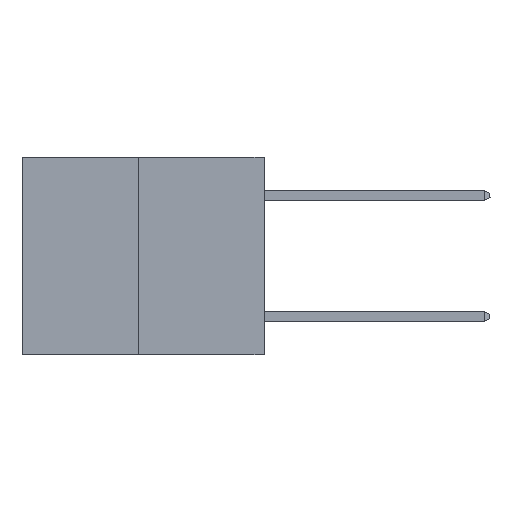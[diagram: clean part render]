
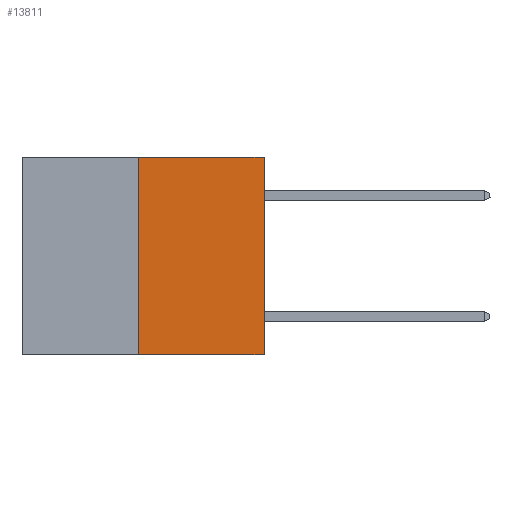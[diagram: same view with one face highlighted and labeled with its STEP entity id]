
A CAD part, left-side view. The second image highlights one B-rep face of the part: STEP entity #13811.
In plain terms, the highlighted planar face has unit normal (-1, 0, 0).
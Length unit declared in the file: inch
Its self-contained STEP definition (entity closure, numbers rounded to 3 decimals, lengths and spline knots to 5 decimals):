
#573 = AXIS2_PLACEMENT_3D ( 'NONE', #8845, #24114, #28576 ) ;
#2399 = EDGE_CURVE ( 'NONE', #14355, #13996, #10141, .T. ) ;
#3822 = LINE ( 'NONE', #12232, #25689 ) ;
#4043 = VECTOR ( 'NONE', #13851, 39.37008 ) ;
#5696 = CARTESIAN_POINT ( 'NONE',  ( 0., 0., 0. ) ) ;
#6281 = VERTEX_POINT ( 'NONE', #5696 ) ;
#8845 = CARTESIAN_POINT ( 'NONE',  ( 0., 0.6, 0. ) ) ;
#8873 = EDGE_LOOP ( 'NONE', ( #11994, #26627, #20147, #11247 ) ) ;
#9110 = CARTESIAN_POINT ( 'NONE',  ( 0., 0., -0.49 ) ) ;
#9445 = VECTOR ( 'NONE', #18754, 39.37008 ) ;
#9467 = FACE_OUTER_BOUND ( 'NONE', #8873, .T. ) ;
#10141 = LINE ( 'NONE', #27451, #9445 ) ;
#11034 = DIRECTION ( 'NONE',  ( 0., -1., 0. ) ) ;
#11247 = ORIENTED_EDGE ( 'NONE', *, *, #27629, .F. ) ;
#11627 = CARTESIAN_POINT ( 'NONE',  ( 0., 0.312, -0.49 ) ) ;
#11994 = ORIENTED_EDGE ( 'NONE', *, *, #18706, .F. ) ;
#12232 = CARTESIAN_POINT ( 'NONE',  ( 0., 0., 0. ) ) ;
#12334 = DIRECTION ( 'NONE',  ( 0., 0., 1. ) ) ;
#13811 = ADVANCED_FACE ( 'NONE', ( #9467 ), #19900, .F. ) ;
#13851 = DIRECTION ( 'NONE',  ( 0., 0., 1. ) ) ;
#13996 = VERTEX_POINT ( 'NONE', #9110 ) ;
#14355 = VERTEX_POINT ( 'NONE', #18412 ) ;
#14682 = VERTEX_POINT ( 'NONE', #25163 ) ;
#15462 = EDGE_CURVE ( 'NONE', #13996, #6281, #3822, .T. ) ;
#15867 = LINE ( 'NONE', #11627, #4043 ) ;
#18412 = CARTESIAN_POINT ( 'NONE',  ( 0., 0.312, -0.49 ) ) ;
#18706 = EDGE_CURVE ( 'NONE', #14355, #14682, #15867, .T. ) ;
#18754 = DIRECTION ( 'NONE',  ( 0., -1., 0. ) ) ;
#19900 = PLANE ( 'NONE',  #573 ) ;
#20147 = ORIENTED_EDGE ( 'NONE', *, *, #15462, .T. ) ;
#24114 = DIRECTION ( 'NONE',  ( 1., 0., 0. ) ) ;
#24460 = CARTESIAN_POINT ( 'NONE',  ( 0., 0.6, 0. ) ) ;
#25163 = CARTESIAN_POINT ( 'NONE',  ( 0., 0.312, 0. ) ) ;
#25689 = VECTOR ( 'NONE', #12334, 39.37008 ) ;
#26627 = ORIENTED_EDGE ( 'NONE', *, *, #2399, .T. ) ;
#27035 = LINE ( 'NONE', #24460, #27406 ) ;
#27406 = VECTOR ( 'NONE', #11034, 39.37008 ) ;
#27451 = CARTESIAN_POINT ( 'NONE',  ( 0., 0.6, -0.49 ) ) ;
#27629 = EDGE_CURVE ( 'NONE', #14682, #6281, #27035, .T. ) ;
#28576 = DIRECTION ( 'NONE',  ( 0., 0., -1. ) ) ;
